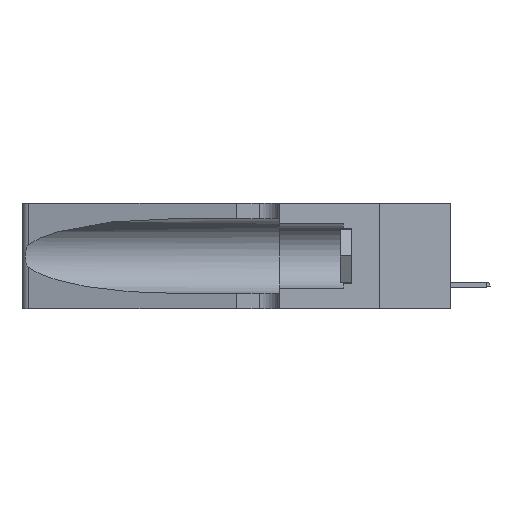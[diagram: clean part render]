
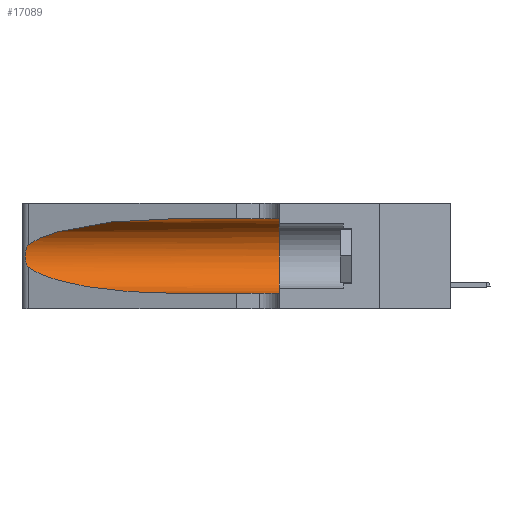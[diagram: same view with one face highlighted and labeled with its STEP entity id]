
A CAD part, left-side view. The second image highlights one B-rep face of the part: STEP entity #17089.
In plain terms, the highlighted cylindrical face has radius 3.308 mm (diameter 6.617 mm), a partial arc.
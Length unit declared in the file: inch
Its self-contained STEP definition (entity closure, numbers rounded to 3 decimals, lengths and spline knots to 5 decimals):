
#140 = AXIS2_PLACEMENT_3D ( 'NONE', #20834, #17173, #19867 ) ;
#543 = VERTEX_POINT ( 'NONE', #43275 ) ;
#677 = CARTESIAN_POINT ( 'NONE',  ( 0.26075, 1.23896, 0.19203 ) ) ;
#1309 = VERTEX_POINT ( 'NONE', #44118 ) ;
#1657 = CARTESIAN_POINT ( 'NONE',  ( 0.26018, 1.23835, 0.19895 ) ) ;
#1877 = DIRECTION ( 'NONE',  ( 0., 0., 1. ) ) ;
#3109 = CARTESIAN_POINT ( 'NONE',  ( 0.1305, 0.72297, 0.05475 ) ) ;
#3581 = CARTESIAN_POINT ( 'NONE',  ( 0.25487, 1.22718, 0.14631 ) ) ;
#4488 = ORIENTED_EDGE ( 'NONE', *, *, #13982, .T. ) ;
#4589 = CARTESIAN_POINT ( 'NONE',  ( 0.25639, 1.23184, 0.21858 ) ) ;
#4600 = DIRECTION ( 'NONE',  ( 0., -1., 0. ) ) ;
#5156 = CARTESIAN_POINT ( 'NONE',  ( 0.1305, 1.61858, 0.05475 ) ) ;
#6237 = CARTESIAN_POINT ( 'NONE',  ( 0.25487, 1.22718, 0.14631 ) ) ;
#8230 = CARTESIAN_POINT ( 'NONE',  ( 0.1305, 1.61858, 0.31525 ) ) ;
#9069 = VERTEX_POINT ( 'NONE', #34208 ) ;
#9676 = FACE_OUTER_BOUND ( 'NONE', #39944, .T. ) ;
#10053 = VECTOR ( 'NONE', #31613, 39.37008 ) ;
#11819 = CARTESIAN_POINT ( 'NONE',  ( 0.25856, 1.23593, 0.16098 ) ) ;
#13655 = ORIENTED_EDGE ( 'NONE', *, *, #42867, .F. ) ;
#13782 = VERTEX_POINT ( 'NONE', #47639 ) ;
#13982 = EDGE_CURVE ( 'NONE', #13782, #37022, #23701, .T. ) ;
#16126 = AXIS2_PLACEMENT_3D ( 'NONE', #24189, #16181, #1877 ) ;
#16181 = DIRECTION ( 'NONE',  ( 0., 1., 0. ) ) ;
#16441 = CARTESIAN_POINT ( 'NONE',  ( 0.25487, 1.22718, 0.14631 ) ) ;
#17089 = ADVANCED_FACE ( 'NONE', ( #9676 ), #39345, .F. ) ;
#17173 = DIRECTION ( 'NONE',  ( 0., -1., 0. ) ) ;
#17470 = CARTESIAN_POINT ( 'NONE',  ( 0.1305, 0.35, 0.05475 ) ) ;
#18144 = ORIENTED_EDGE ( 'NONE', *, *, #29351, .T. ) ;
#18677 = CARTESIAN_POINT ( 'NONE',  ( 0.18966, 0.96281, 0.31525 ) ) ;
#19123 = CARTESIAN_POINT ( 'NONE',  ( 0.25555, 1.22993, 0.14849 ) ) ;
#19852 = CARTESIAN_POINT ( 'NONE',  ( 0.25487, 1.22718, 0.22369 ) ) ;
#19867 = DIRECTION ( 'NONE',  ( 0., 0., -1. ) ) ;
#20093 = CARTESIAN_POINT ( 'NONE',  ( 0.25787, 1.23484, 0.2124 ) ) ;
#20229 = ORIENTED_EDGE ( 'NONE', *, *, #39849, .T. ) ;
#20834 = CARTESIAN_POINT ( 'NONE',  ( 0.1305, 1.61858, 0.185 ) ) ;
#23701 = B_SPLINE_CURVE_WITH_KNOTS ( 'NONE', 3,
 ( #19852, #26656, #4589, #20093, #34706, #1657, #677, #31284, #38113, #11819, #23986, #46160, #19123, #16441 ),
 .UNSPECIFIED., .F., .F.,
 ( 4, 2, 2, 2, 2, 2, 4 ),
 ( 0., 0.00027, 0.00053, 0.00107, 0.0016, 0.00187, 0.00214 ),
 .UNSPECIFIED. ) ;
#23973 = VERTEX_POINT ( 'NONE', #17470 ) ;
#23986 = CARTESIAN_POINT ( 'NONE',  ( 0.25789, 1.23486, 0.15765 ) ) ;
#24189 = CARTESIAN_POINT ( 'NONE',  ( 0.1305, 0.35, 0.185 ) ) ;
#26656 = CARTESIAN_POINT ( 'NONE',  ( 0.25555, 1.22994, 0.2215 ) ) ;
#28918 = VECTOR ( 'NONE', #4600, 39.37008 ) ;
#29351 = EDGE_CURVE ( 'NONE', #9069, #23973, #35265, .T. ) ;
#29864 = ORIENTED_EDGE ( 'NONE', *, *, #35131, .F. ) ;
#30581 = CARTESIAN_POINT ( 'NONE',  ( 0.1305, 0.72297, 0.31525 ) ) ;
#31284 = CARTESIAN_POINT ( 'NONE',  ( 0.26075, 1.23896, 0.178 ) ) ;
#31613 = DIRECTION ( 'NONE',  ( 0., -1., 0. ) ) ;
#32262 =( BOUNDED_CURVE ( )  B_SPLINE_CURVE ( 3, ( #3581, #36379, #37101, #3109 ),
 .UNSPECIFIED., .F., .F. ) 
 B_SPLINE_CURVE_WITH_KNOTS ( ( 4, 4 ),
 ( 3.44316, 4.71239 ),
 .UNSPECIFIED. ) 
 CURVE ( )  GEOMETRIC_REPRESENTATION_ITEM ( )  RATIONAL_B_SPLINE_CURVE ( ( 1., 0.87, 0.87, 1. ) ) 
 REPRESENTATION_ITEM ( '' )  );
#34208 = CARTESIAN_POINT ( 'NONE',  ( 0.1305, 0.72297, 0.05475 ) ) ;
#34706 = CARTESIAN_POINT ( 'NONE',  ( 0.25854, 1.2359, 0.20912 ) ) ;
#35131 = EDGE_CURVE ( 'NONE', #543, #1309, #41539, .T. ) ;
#35265 = LINE ( 'NONE', #5156, #10053 ) ;
#35592 = CIRCLE ( 'NONE', #16126, 0.13025 ) ;
#36379 = CARTESIAN_POINT ( 'NONE',  ( 0.2373, 1.15595, 0.08982 ) ) ;
#37022 = VERTEX_POINT ( 'NONE', #6237 ) ;
#37101 = CARTESIAN_POINT ( 'NONE',  ( 0.18966, 0.96281, 0.05475 ) ) ;
#37227 =( BOUNDED_CURVE ( )  B_SPLINE_CURVE ( 3, ( #30581, #18677, #41811, #38155 ),
 .UNSPECIFIED., .F., .F. ) 
 B_SPLINE_CURVE_WITH_KNOTS ( ( 4, 4 ),
 ( 1.5708, 2.84003 ),
 .UNSPECIFIED. ) 
 CURVE ( )  GEOMETRIC_REPRESENTATION_ITEM ( )  RATIONAL_B_SPLINE_CURVE ( ( 1., 0.87, 0.87, 1. ) ) 
 REPRESENTATION_ITEM ( '' )  );
#38113 = CARTESIAN_POINT ( 'NONE',  ( 0.26017, 1.23833, 0.17102 ) ) ;
#38155 = CARTESIAN_POINT ( 'NONE',  ( 0.25487, 1.22718, 0.22369 ) ) ;
#39345 = CYLINDRICAL_SURFACE ( 'NONE', #140, 0.13025 ) ;
#39849 = EDGE_CURVE ( 'NONE', #37022, #9069, #32262, .T. ) ;
#39944 = EDGE_LOOP ( 'NONE', ( #43342, #4488, #20229, #18144, #13655, #29864 ) ) ;
#41539 = LINE ( 'NONE', #8230, #28918 ) ;
#41811 = CARTESIAN_POINT ( 'NONE',  ( 0.2373, 1.15595, 0.28018 ) ) ;
#42867 = EDGE_CURVE ( 'NONE', #1309, #23973, #35592, .T. ) ;
#43275 = CARTESIAN_POINT ( 'NONE',  ( 0.1305, 0.72297, 0.31525 ) ) ;
#43342 = ORIENTED_EDGE ( 'NONE', *, *, #43454, .T. ) ;
#43454 = EDGE_CURVE ( 'NONE', #543, #13782, #37227, .T. ) ;
#44118 = CARTESIAN_POINT ( 'NONE',  ( 0.1305, 0.35, 0.31525 ) ) ;
#46160 = CARTESIAN_POINT ( 'NONE',  ( 0.25639, 1.23186, 0.15144 ) ) ;
#47639 = CARTESIAN_POINT ( 'NONE',  ( 0.25487, 1.22718, 0.22369 ) ) ;
